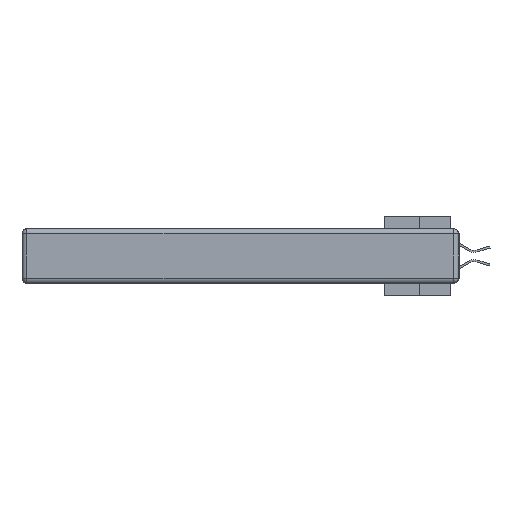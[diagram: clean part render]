
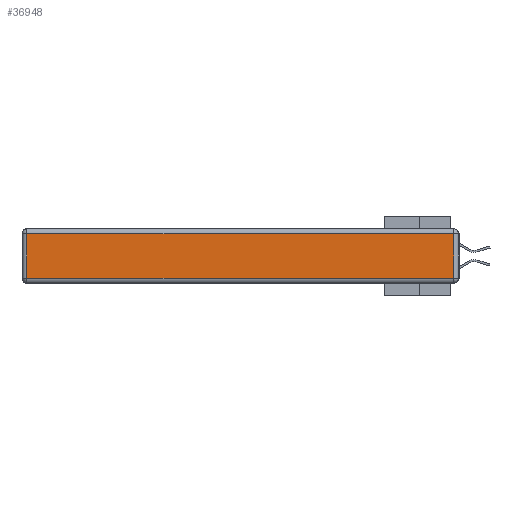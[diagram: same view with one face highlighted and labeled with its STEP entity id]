
A CAD part, left-side view. The second image highlights one B-rep face of the part: STEP entity #36948.
In plain terms, the highlighted planar face has unit normal (-1, 0, 0).
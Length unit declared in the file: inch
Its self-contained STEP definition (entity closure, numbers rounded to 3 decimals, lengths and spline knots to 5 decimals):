
#110 = ORIENTED_EDGE ( 'NONE', *, *, #6650, .T. ) ;
#967 = LINE ( 'NONE', #12713, #33406 ) ;
#4484 = DIRECTION ( 'NONE',  ( -1., 0., 0. ) ) ;
#6641 = PLANE ( 'NONE',  #29571 ) ;
#6650 = EDGE_CURVE ( 'NONE', #10427, #24123, #10715, .T. ) ;
#7458 = CARTESIAN_POINT ( 'NONE',  ( 0., 0.03, -0.313 ) ) ;
#10427 = VERTEX_POINT ( 'NONE', #37680 ) ;
#10715 = LINE ( 'NONE', #22112, #12377 ) ;
#12377 = VECTOR ( 'NONE', #18983, 39.37008 ) ;
#12713 = CARTESIAN_POINT ( 'NONE',  ( 0., 0.03, -0.343 ) ) ;
#13285 = DIRECTION ( 'NONE',  ( 0., 0., 1. ) ) ;
#14451 = VECTOR ( 'NONE', #28441, 39.37008 ) ;
#18629 = CARTESIAN_POINT ( 'NONE',  ( 0., 0., -0.343 ) ) ;
#18983 = DIRECTION ( 'NONE',  ( 0., 0., -1. ) ) ;
#19369 = EDGE_CURVE ( 'NONE', #26986, #10427, #37857, .T. ) ;
#19454 = VECTOR ( 'NONE', #23157, 39.37008 ) ;
#19652 = LINE ( 'NONE', #34907, #14451 ) ;
#21561 = FACE_OUTER_BOUND ( 'NONE', #34556, .T. ) ;
#22112 = CARTESIAN_POINT ( 'NONE',  ( 0., 2.72, -0.343 ) ) ;
#22549 = EDGE_CURVE ( 'NONE', #30929, #26986, #967, .T. ) ;
#22757 = ORIENTED_EDGE ( 'NONE', *, *, #22549, .T. ) ;
#23157 = DIRECTION ( 'NONE',  ( 0., 1., 0. ) ) ;
#24123 = VERTEX_POINT ( 'NONE', #31738 ) ;
#24557 = ORIENTED_EDGE ( 'NONE', *, *, #19369, .T. ) ;
#26502 = ORIENTED_EDGE ( 'NONE', *, *, #27631, .T. ) ;
#26986 = VERTEX_POINT ( 'NONE', #28970 ) ;
#27631 = EDGE_CURVE ( 'NONE', #24123, #30929, #19652, .T. ) ;
#28441 = DIRECTION ( 'NONE',  ( 0., -1., 0. ) ) ;
#28970 = CARTESIAN_POINT ( 'NONE',  ( 0., 0.03, -0.03 ) ) ;
#29571 = AXIS2_PLACEMENT_3D ( 'NONE', #18629, #4484, #34057 ) ;
#30929 = VERTEX_POINT ( 'NONE', #7458 ) ;
#31738 = CARTESIAN_POINT ( 'NONE',  ( 0., 2.72, -0.313 ) ) ;
#31759 = CARTESIAN_POINT ( 'NONE',  ( 0., 2.75, -0.03 ) ) ;
#33406 = VECTOR ( 'NONE', #13285, 39.37008 ) ;
#34057 = DIRECTION ( 'NONE',  ( 0., 0., 1. ) ) ;
#34556 = EDGE_LOOP ( 'NONE', ( #26502, #22757, #24557, #110 ) ) ;
#34907 = CARTESIAN_POINT ( 'NONE',  ( 0., 0., -0.313 ) ) ;
#36948 = ADVANCED_FACE ( 'NONE', ( #21561 ), #6641, .T. ) ;
#37680 = CARTESIAN_POINT ( 'NONE',  ( 0., 2.72, -0.03 ) ) ;
#37857 = LINE ( 'NONE', #31759, #19454 ) ;
